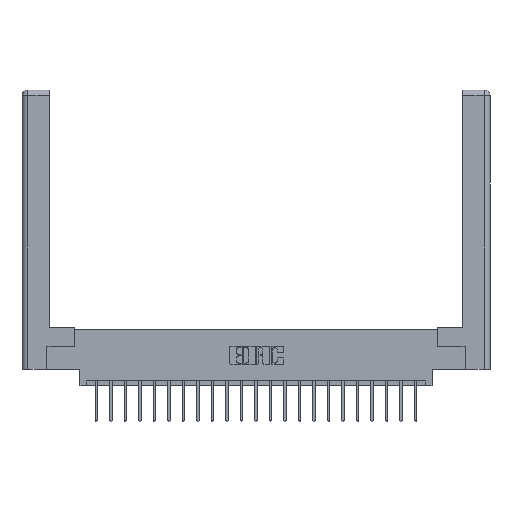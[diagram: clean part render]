
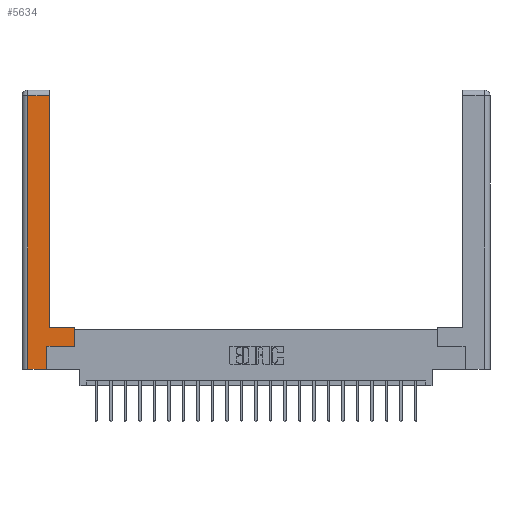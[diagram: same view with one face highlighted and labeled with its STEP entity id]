
A CAD part, top view. The second image highlights one B-rep face of the part: STEP entity #5634.
In plain terms, the highlighted planar face has unit normal (0, 0, 1).
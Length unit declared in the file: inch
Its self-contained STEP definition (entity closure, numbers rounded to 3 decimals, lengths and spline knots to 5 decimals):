
#83 = VECTOR ( 'NONE', #5716, 39.37008 ) ;
#138 = EDGE_CURVE ( 'NONE', #17586, #4957, #9539, .T. ) ;
#171 = DIRECTION ( 'NONE',  ( -1., 0., 0. ) ) ;
#1064 = VERTEX_POINT ( 'NONE', #20567 ) ;
#1950 = CARTESIAN_POINT ( 'NONE',  ( 0.265, 0.245, 0. ) ) ;
#1993 = EDGE_CURVE ( 'NONE', #22321, #10151, #17346, .T. ) ;
#2083 = ORIENTED_EDGE ( 'NONE', *, *, #21782, .T. ) ;
#2890 = LINE ( 'NONE', #1950, #83 ) ;
#3213 = CARTESIAN_POINT ( 'NONE',  ( 0.565, 0.45, 0. ) ) ;
#3451 = ORIENTED_EDGE ( 'NONE', *, *, #13178, .T. ) ;
#3501 = ORIENTED_EDGE ( 'NONE', *, *, #1993, .T. ) ;
#3514 = CARTESIAN_POINT ( 'NONE',  ( 0.265, 0.245, 0. ) ) ;
#3626 = EDGE_CURVE ( 'NONE', #1064, #22321, #10607, .T. ) ;
#3696 = DIRECTION ( 'NONE',  ( 0., 1., 0. ) ) ;
#4200 = VECTOR ( 'NONE', #14773, 39.37008 ) ;
#4709 = CARTESIAN_POINT ( 'NONE',  ( 0.265, 0., 0. ) ) ;
#4957 = VERTEX_POINT ( 'NONE', #3213 ) ;
#5537 = DIRECTION ( 'NONE',  ( 0., 0., -1. ) ) ;
#5615 = EDGE_LOOP ( 'NONE', ( #3451, #22090, #3501, #17428, #13468, #2083, #8887, #12682 ) ) ;
#5634 = ADVANCED_FACE ( 'NONE', ( #6045 ), #10863, .F. ) ;
#5716 = DIRECTION ( 'NONE',  ( 0., 1., 0. ) ) ;
#6045 = FACE_OUTER_BOUND ( 'NONE', #5615, .T. ) ;
#6063 = LINE ( 'NONE', #7018, #14745 ) ;
#6149 = AXIS2_PLACEMENT_3D ( 'NONE', #16241, #5537, #171 ) ;
#6414 = VERTEX_POINT ( 'NONE', #4709 ) ;
#6557 = VECTOR ( 'NONE', #9336, 39.37008 ) ;
#6843 = CARTESIAN_POINT ( 'NONE',  ( 0.565, 0.245, 0. ) ) ;
#6902 = CARTESIAN_POINT ( 'NONE',  ( 0.0615, 0., 0. ) ) ;
#7018 = CARTESIAN_POINT ( 'NONE',  ( 0.265, 0., 0. ) ) ;
#7482 = DIRECTION ( 'NONE',  ( -1., 0., 0. ) ) ;
#7657 = CARTESIAN_POINT ( 'NONE',  ( 0.0615, 0., 0. ) ) ;
#7992 = CARTESIAN_POINT ( 'NONE',  ( 0.0615, 2.94, 0. ) ) ;
#8646 = VECTOR ( 'NONE', #7482, 39.37008 ) ;
#8887 = ORIENTED_EDGE ( 'NONE', *, *, #138, .T. ) ;
#9336 = DIRECTION ( 'NONE',  ( 1., 0., 0. ) ) ;
#9539 = LINE ( 'NONE', #14381, #14847 ) ;
#9632 = LINE ( 'NONE', #11120, #6557 ) ;
#10151 = VERTEX_POINT ( 'NONE', #7657 ) ;
#10607 = LINE ( 'NONE', #16434, #8646 ) ;
#10686 = DIRECTION ( 'NONE',  ( 1., 0., 0. ) ) ;
#10863 = PLANE ( 'NONE',  #6149 ) ;
#10866 = CARTESIAN_POINT ( 'NONE',  ( 0.295, 0.45, 0. ) ) ;
#11040 = VECTOR ( 'NONE', #14954, 39.37008 ) ;
#11120 = CARTESIAN_POINT ( 'NONE',  ( 0.565, 0.245, 0. ) ) ;
#12025 = EDGE_CURVE ( 'NONE', #10151, #6414, #6063, .T. ) ;
#12158 = LINE ( 'NONE', #22223, #11040 ) ;
#12497 = VERTEX_POINT ( 'NONE', #3514 ) ;
#12682 = ORIENTED_EDGE ( 'NONE', *, *, #17989, .T. ) ;
#13178 = EDGE_CURVE ( 'NONE', #17204, #1064, #12158, .T. ) ;
#13468 = ORIENTED_EDGE ( 'NONE', *, *, #15787, .T. ) ;
#14381 = CARTESIAN_POINT ( 'NONE',  ( 0.565, 0.45, 0. ) ) ;
#14745 = VECTOR ( 'NONE', #10686, 39.37008 ) ;
#14773 = DIRECTION ( 'NONE',  ( -1., 0., 0. ) ) ;
#14847 = VECTOR ( 'NONE', #3696, 39.37008 ) ;
#14954 = DIRECTION ( 'NONE',  ( 0., 1., 0. ) ) ;
#15787 = EDGE_CURVE ( 'NONE', #6414, #12497, #2890, .T. ) ;
#15915 = LINE ( 'NONE', #16551, #4200 ) ;
#16241 = CARTESIAN_POINT ( 'NONE',  ( 0., 0., 0. ) ) ;
#16434 = CARTESIAN_POINT ( 'NONE',  ( 0.0615, 2.94, 0. ) ) ;
#16551 = CARTESIAN_POINT ( 'NONE',  ( 0.295, 0.45, 0. ) ) ;
#17194 = DIRECTION ( 'NONE',  ( 0., -1., 0. ) ) ;
#17204 = VERTEX_POINT ( 'NONE', #10866 ) ;
#17346 = LINE ( 'NONE', #6902, #17613 ) ;
#17428 = ORIENTED_EDGE ( 'NONE', *, *, #12025, .T. ) ;
#17586 = VERTEX_POINT ( 'NONE', #6843 ) ;
#17613 = VECTOR ( 'NONE', #17194, 39.37008 ) ;
#17989 = EDGE_CURVE ( 'NONE', #4957, #17204, #15915, .T. ) ;
#20567 = CARTESIAN_POINT ( 'NONE',  ( 0.295, 2.94, 0. ) ) ;
#21782 = EDGE_CURVE ( 'NONE', #12497, #17586, #9632, .T. ) ;
#22090 = ORIENTED_EDGE ( 'NONE', *, *, #3626, .T. ) ;
#22223 = CARTESIAN_POINT ( 'NONE',  ( 0.295, 3., 0. ) ) ;
#22321 = VERTEX_POINT ( 'NONE', #7992 ) ;
